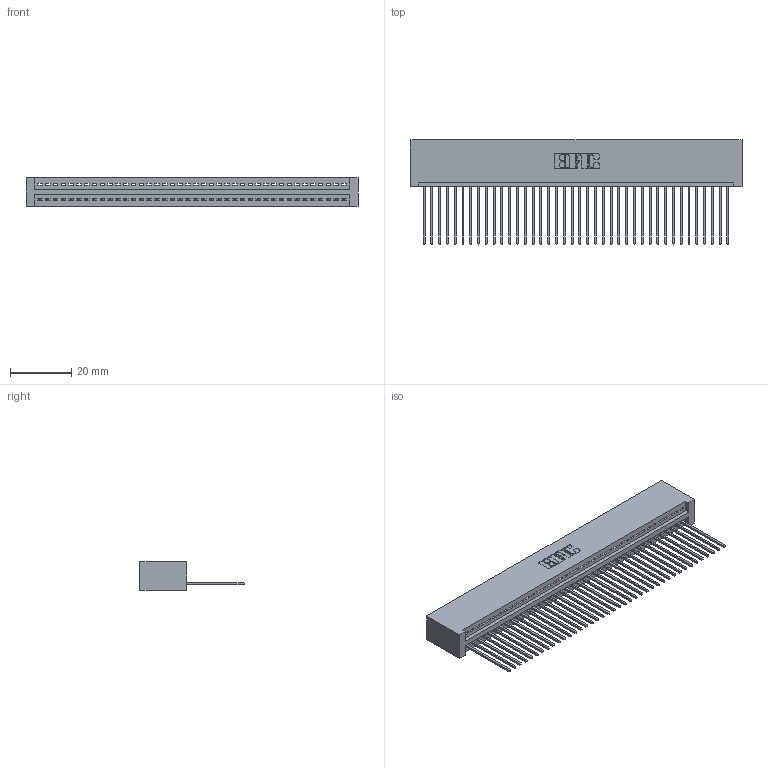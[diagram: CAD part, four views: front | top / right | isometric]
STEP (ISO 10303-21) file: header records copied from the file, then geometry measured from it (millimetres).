
FILE_DESCRIPTION (( 'STEP AP203' ), '1' );
FILE_NAME ('345-040-541-101.STEP', '2018-09-05T03:16:01', ( '' ), ( '' ), 'SwSTEP 2.0', 'SolidWorks 2016', '' );
FILE_SCHEMA (( 'CONFIG_CONTROL_DESIGN' ));
Length unit declared in the file: inch
Products named in the file (3): 345 Part_No Mounting Lugs; 345-292-001_345-293-141; 345-040-541-101
Assembly tree (41 placements, depth 2):
  345-040-541-101
    345 Part_No Mounting Lugs
    345-292-001_345-293-141  x40
Bounding box: 108.2 x 33.96 x 9.4 mm (x, y, z)
Volume: 10977.3 mm3; surface area: 15527.4 mm2
Topology: 41 solids, 41 shells, 2438 faces, 7357 edges, 4850 vertices
Faces by surface type: plane 1676, cylinder 762
Entity records: 30115 total; most frequent: CARTESIAN_POINT 5224, ORIENTED_EDGE 5198, DIRECTION 4559, EDGE_CURVE 2599, LINE 2315, VECTOR 2315, VERTEX_POINT 1730, AXIS2_PLACEMENT_3D 1122
